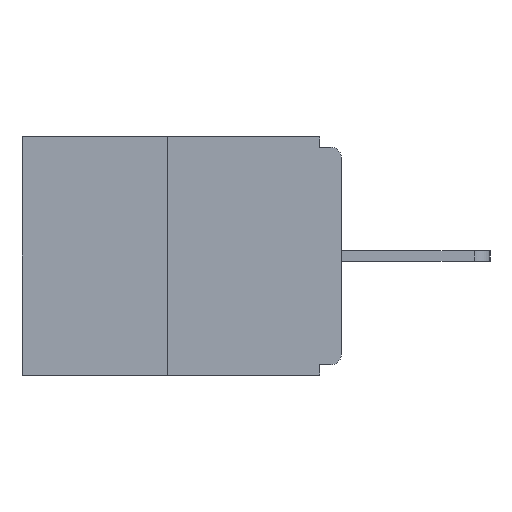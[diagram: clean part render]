
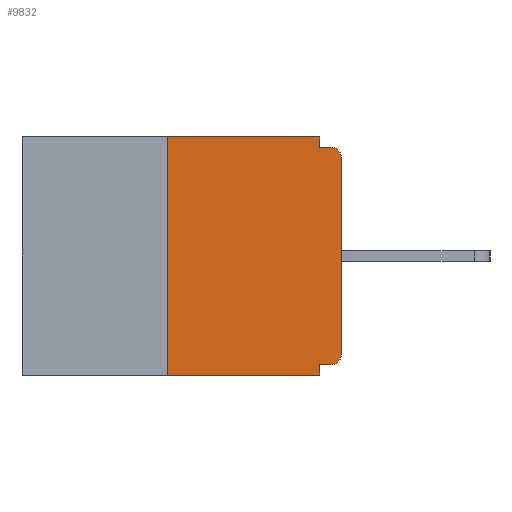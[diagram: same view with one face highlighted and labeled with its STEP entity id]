
A CAD part, left-side view. The second image highlights one B-rep face of the part: STEP entity #9832.
In plain terms, the highlighted planar face has unit normal (-1, 0, 0).
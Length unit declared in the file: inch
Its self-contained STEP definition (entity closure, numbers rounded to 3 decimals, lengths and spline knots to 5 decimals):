
#206 = EDGE_CURVE ( 'NONE', #12297, #3532, #3831, .T. ) ;
#222 = CARTESIAN_POINT ( 'NONE',  ( 0., 0.031, 0. ) ) ;
#289 = AXIS2_PLACEMENT_3D ( 'NONE', #14767, #15020, #4401 ) ;
#727 = VECTOR ( 'NONE', #16793, 39.37008 ) ;
#1319 = LINE ( 'NONE', #13241, #11261 ) ;
#1398 = AXIS2_PLACEMENT_3D ( 'NONE', #13962, #7325, #12858 ) ;
#1465 = VERTEX_POINT ( 'NONE', #4645 ) ;
#1618 = VERTEX_POINT ( 'NONE', #2044 ) ;
#2044 = CARTESIAN_POINT ( 'NONE',  ( 0., 0.015, -0.328 ) ) ;
#2309 = PLANE ( 'NONE',  #1398 ) ;
#2721 = DIRECTION ( 'NONE',  ( 0., -1., 0. ) ) ;
#2889 = ORIENTED_EDGE ( 'NONE', *, *, #8980, .F. ) ;
#3037 = CARTESIAN_POINT ( 'NONE',  ( 0., 0., 0. ) ) ;
#3336 = DIRECTION ( 'NONE',  ( 0., -1., 0. ) ) ;
#3532 = VERTEX_POINT ( 'NONE', #5352 ) ;
#3559 = VERTEX_POINT ( 'NONE', #11684 ) ;
#3831 = LINE ( 'NONE', #7734, #727 ) ;
#3861 = VERTEX_POINT ( 'NONE', #10271 ) ;
#4217 = VERTEX_POINT ( 'NONE', #16873 ) ;
#4369 = VECTOR ( 'NONE', #2721, 39.37008 ) ;
#4401 = DIRECTION ( 'NONE',  ( 0., 0., -1. ) ) ;
#4645 = CARTESIAN_POINT ( 'NONE',  ( 0., 0.031, 0. ) ) ;
#4808 = FACE_OUTER_BOUND ( 'NONE', #11908, .T. ) ;
#4979 = CIRCLE ( 'NONE', #289, 0.015 ) ;
#5113 = CARTESIAN_POINT ( 'NONE',  ( 0., 0.25, -0.343 ) ) ;
#5137 = LINE ( 'NONE', #10432, #4369 ) ;
#5352 = CARTESIAN_POINT ( 'NONE',  ( 0., 0.25, 0. ) ) ;
#5521 = CARTESIAN_POINT ( 'NONE',  ( 0., 0.031, -0.343 ) ) ;
#5723 = LINE ( 'NONE', #11002, #12602 ) ;
#5797 = EDGE_CURVE ( 'NONE', #6384, #9308, #5984, .T. ) ;
#5878 = CARTESIAN_POINT ( 'NONE',  ( 0., 0., -0.03 ) ) ;
#5969 = DIRECTION ( 'NONE',  ( 0., -1., 0. ) ) ;
#5984 = LINE ( 'NONE', #3037, #15918 ) ;
#6042 = ORIENTED_EDGE ( 'NONE', *, *, #8734, .F. ) ;
#6248 = ORIENTED_EDGE ( 'NONE', *, *, #12214, .F. ) ;
#6384 = VERTEX_POINT ( 'NONE', #15030 ) ;
#6594 = ORIENTED_EDGE ( 'NONE', *, *, #5797, .T. ) ;
#6703 = DIRECTION ( 'NONE',  ( 0., 0., -1. ) ) ;
#6900 = ORIENTED_EDGE ( 'NONE', *, *, #13892, .T. ) ;
#6962 = LINE ( 'NONE', #222, #13264 ) ;
#7188 = CARTESIAN_POINT ( 'NONE',  ( 0., 0., -0.015 ) ) ;
#7325 = DIRECTION ( 'NONE',  ( 1., 0., 0. ) ) ;
#7501 = LINE ( 'NONE', #15426, #13002 ) ;
#7734 = CARTESIAN_POINT ( 'NONE',  ( 0., 0.25, 0. ) ) ;
#8065 = VERTEX_POINT ( 'NONE', #5521 ) ;
#8322 = DIRECTION ( 'NONE',  ( 0., 0., 1. ) ) ;
#8734 = EDGE_CURVE ( 'NONE', #3532, #1465, #7501, .T. ) ;
#8980 = EDGE_CURVE ( 'NONE', #1465, #3861, #6962, .T. ) ;
#9061 = ORIENTED_EDGE ( 'NONE', *, *, #12462, .F. ) ;
#9226 = ORIENTED_EDGE ( 'NONE', *, *, #9386, .T. ) ;
#9308 = VERTEX_POINT ( 'NONE', #5878 ) ;
#9386 = EDGE_CURVE ( 'NONE', #1618, #6384, #4979, .T. ) ;
#9609 = LINE ( 'NONE', #7188, #13150 ) ;
#9832 = ADVANCED_FACE ( 'NONE', ( #4808 ), #2309, .F. ) ;
#10013 = ORIENTED_EDGE ( 'NONE', *, *, #14956, .F. ) ;
#10128 = DIRECTION ( 'NONE',  ( -1., 0., 0. ) ) ;
#10271 = CARTESIAN_POINT ( 'NONE',  ( 0., 0.031, -0.015 ) ) ;
#10389 = DIRECTION ( 'NONE',  ( 0., 0., -1. ) ) ;
#10432 = CARTESIAN_POINT ( 'NONE',  ( 0., 0.46, -0.343 ) ) ;
#10834 = ORIENTED_EDGE ( 'NONE', *, *, #206, .F. ) ;
#11002 = CARTESIAN_POINT ( 'NONE',  ( 0., 0., -0.328 ) ) ;
#11261 = VECTOR ( 'NONE', #15818, 39.37008 ) ;
#11682 = CARTESIAN_POINT ( 'NONE',  ( 0., 0.015, -0.03 ) ) ;
#11684 = CARTESIAN_POINT ( 'NONE',  ( 0., 0.015, -0.015 ) ) ;
#11908 = EDGE_LOOP ( 'NONE', ( #6042, #10834, #12687, #10013, #6248, #9226, #6594, #6900, #9061, #2889 ) ) ;
#12214 = EDGE_CURVE ( 'NONE', #1618, #4217, #5723, .T. ) ;
#12297 = VERTEX_POINT ( 'NONE', #5113 ) ;
#12462 = EDGE_CURVE ( 'NONE', #3861, #3559, #9609, .T. ) ;
#12602 = VECTOR ( 'NONE', #13664, 39.37008 ) ;
#12687 = ORIENTED_EDGE ( 'NONE', *, *, #14605, .T. ) ;
#12858 = DIRECTION ( 'NONE',  ( 0., 0., -1. ) ) ;
#13002 = VECTOR ( 'NONE', #3336, 39.37008 ) ;
#13150 = VECTOR ( 'NONE', #5969, 39.37008 ) ;
#13241 = CARTESIAN_POINT ( 'NONE',  ( 0., 0.031, -0.343 ) ) ;
#13264 = VECTOR ( 'NONE', #6703, 39.37008 ) ;
#13445 = CIRCLE ( 'NONE', #15655, 0.015 ) ;
#13664 = DIRECTION ( 'NONE',  ( 0., 1., 0. ) ) ;
#13892 = EDGE_CURVE ( 'NONE', #9308, #3559, #13445, .T. ) ;
#13962 = CARTESIAN_POINT ( 'NONE',  ( 0., 0.46, 0. ) ) ;
#14605 = EDGE_CURVE ( 'NONE', #12297, #8065, #5137, .T. ) ;
#14767 = CARTESIAN_POINT ( 'NONE',  ( 0., 0.015, -0.313 ) ) ;
#14956 = EDGE_CURVE ( 'NONE', #4217, #8065, #1319, .T. ) ;
#15020 = DIRECTION ( 'NONE',  ( -1., 0., 0. ) ) ;
#15030 = CARTESIAN_POINT ( 'NONE',  ( 0., 0., -0.313 ) ) ;
#15426 = CARTESIAN_POINT ( 'NONE',  ( 0., 0.46, 0. ) ) ;
#15655 = AXIS2_PLACEMENT_3D ( 'NONE', #11682, #10128, #10389 ) ;
#15818 = DIRECTION ( 'NONE',  ( 0., 0., -1. ) ) ;
#15918 = VECTOR ( 'NONE', #8322, 39.37008 ) ;
#16793 = DIRECTION ( 'NONE',  ( 0., 0., 1. ) ) ;
#16873 = CARTESIAN_POINT ( 'NONE',  ( 0., 0.031, -0.328 ) ) ;
